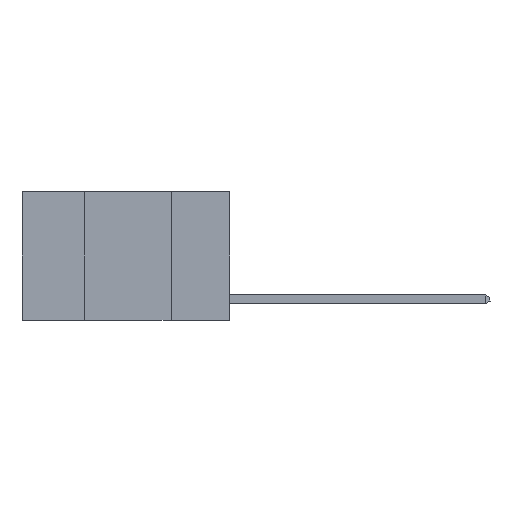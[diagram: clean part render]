
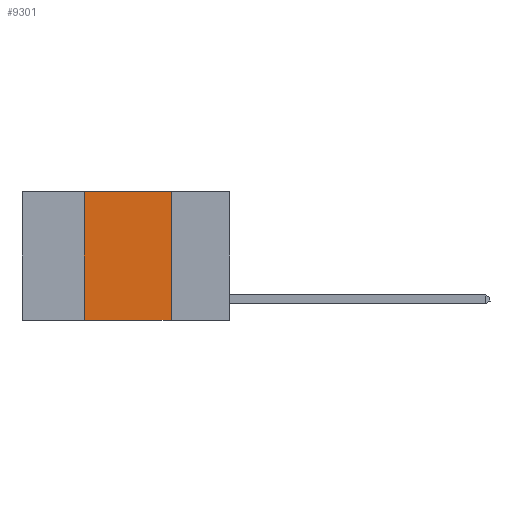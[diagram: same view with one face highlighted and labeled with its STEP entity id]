
A CAD part, left-side view. The second image highlights one B-rep face of the part: STEP entity #9301.
In plain terms, the highlighted planar face has unit normal (-1, 0, 0).
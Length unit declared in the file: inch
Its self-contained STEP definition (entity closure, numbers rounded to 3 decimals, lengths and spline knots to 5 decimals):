
#48 = CARTESIAN_POINT ( 'NONE',  ( 0., 0.42, 0. ) ) ;
#1258 = VECTOR ( 'NONE', #5799, 39.37008 ) ;
#1375 = ORIENTED_EDGE ( 'NONE', *, *, #5527, .F. ) ;
#3201 = LINE ( 'NONE', #48, #13756 ) ;
#5527 = EDGE_CURVE ( 'NONE', #17665, #14496, #11815, .T. ) ;
#5799 = DIRECTION ( 'NONE',  ( 0., -1., 0. ) ) ;
#6553 = EDGE_CURVE ( 'NONE', #14496, #19327, #13336, .T. ) ;
#6759 = DIRECTION ( 'NONE',  ( 0., 0., 1. ) ) ;
#7728 = EDGE_CURVE ( 'NONE', #14517, #19327, #8524, .T. ) ;
#8524 = LINE ( 'NONE', #10874, #19347 ) ;
#9082 = CARTESIAN_POINT ( 'NONE',  ( 0., 0.17, 0. ) ) ;
#9301 = ADVANCED_FACE ( 'NONE', ( #9324 ), #12029, .F. ) ;
#9324 = FACE_OUTER_BOUND ( 'NONE', #16647, .T. ) ;
#9863 = CARTESIAN_POINT ( 'NONE',  ( 0., 0.6, 0. ) ) ;
#9945 = ORIENTED_EDGE ( 'NONE', *, *, #7728, .T. ) ;
#10713 = AXIS2_PLACEMENT_3D ( 'NONE', #15420, #17121, #18811 ) ;
#10874 = CARTESIAN_POINT ( 'NONE',  ( 0., 0.6, -0.37 ) ) ;
#11495 = VECTOR ( 'NONE', #20838, 39.37008 ) ;
#11815 = LINE ( 'NONE', #9863, #1258 ) ;
#12029 = PLANE ( 'NONE',  #10713 ) ;
#13050 = ORIENTED_EDGE ( 'NONE', *, *, #19308, .F. ) ;
#13336 = LINE ( 'NONE', #9082, #11495 ) ;
#13756 = VECTOR ( 'NONE', #6759, 39.37008 ) ;
#14496 = VERTEX_POINT ( 'NONE', #15934 ) ;
#14517 = VERTEX_POINT ( 'NONE', #19319 ) ;
#15420 = CARTESIAN_POINT ( 'NONE',  ( 0., 0.6, 0. ) ) ;
#15934 = CARTESIAN_POINT ( 'NONE',  ( 0., 0.17, 0. ) ) ;
#16647 = EDGE_LOOP ( 'NONE', ( #20078, #1375, #13050, #9945 ) ) ;
#17037 = CARTESIAN_POINT ( 'NONE',  ( 0., 0.42, 0. ) ) ;
#17121 = DIRECTION ( 'NONE',  ( 1., 0., 0. ) ) ;
#17665 = VERTEX_POINT ( 'NONE', #17037 ) ;
#18811 = DIRECTION ( 'NONE',  ( 0., 0., -1. ) ) ;
#19308 = EDGE_CURVE ( 'NONE', #14517, #17665, #3201, .T. ) ;
#19319 = CARTESIAN_POINT ( 'NONE',  ( 0., 0.42, -0.37 ) ) ;
#19327 = VERTEX_POINT ( 'NONE', #21733 ) ;
#19347 = VECTOR ( 'NONE', #21161, 39.37008 ) ;
#20078 = ORIENTED_EDGE ( 'NONE', *, *, #6553, .F. ) ;
#20838 = DIRECTION ( 'NONE',  ( 0., 0., -1. ) ) ;
#21161 = DIRECTION ( 'NONE',  ( 0., -1., 0. ) ) ;
#21733 = CARTESIAN_POINT ( 'NONE',  ( 0., 0.17, -0.37 ) ) ;
